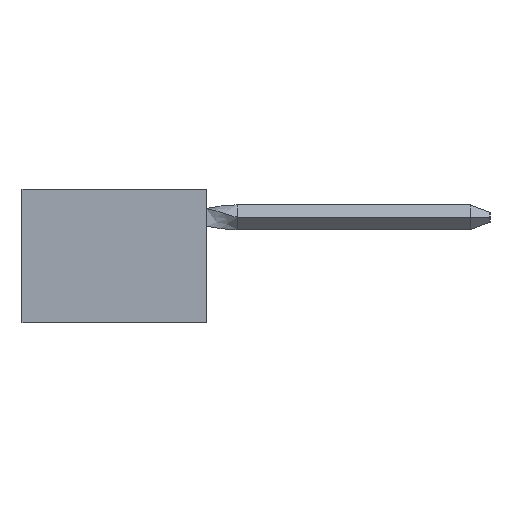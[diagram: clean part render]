
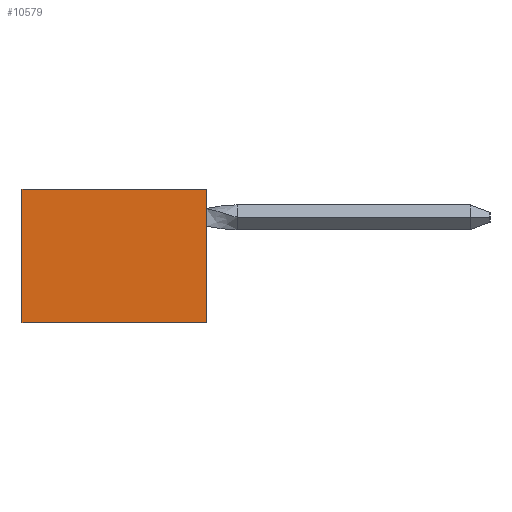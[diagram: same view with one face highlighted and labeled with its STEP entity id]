
A CAD part, left-side view. The second image highlights one B-rep face of the part: STEP entity #10579.
In plain terms, the highlighted planar face has unit normal (-1, 0, 0).
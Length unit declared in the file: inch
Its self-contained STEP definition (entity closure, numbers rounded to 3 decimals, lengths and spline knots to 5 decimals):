
#341 = LINE ( 'NONE', #5239, #14562 ) ;
#389 = LINE ( 'NONE', #11272, #28761 ) ;
#929 = PLANE ( 'NONE',  #28540 ) ;
#1542 = LINE ( 'NONE', #12609, #11297 ) ;
#4967 = VERTEX_POINT ( 'NONE', #35249 ) ;
#5239 = CARTESIAN_POINT ( 'NONE',  ( 0.298, 0., -0.343 ) ) ;
#5421 = EDGE_CURVE ( 'NONE', #27252, #29198, #389, .T. ) ;
#5598 = CARTESIAN_POINT ( 'NONE',  ( 0.298, 0.473, 0. ) ) ;
#7021 = CARTESIAN_POINT ( 'NONE',  ( 0.298, 0., 0. ) ) ;
#7313 = LINE ( 'NONE', #35291, #29466 ) ;
#9545 = EDGE_CURVE ( 'NONE', #16041, #27252, #1542, .T. ) ;
#10579 = ADVANCED_FACE ( 'NONE', ( #16104 ), #929, .F. ) ;
#10687 = DIRECTION ( 'NONE',  ( 0., 0., 1. ) ) ;
#11255 = ORIENTED_EDGE ( 'NONE', *, *, #5421, .T. ) ;
#11272 = CARTESIAN_POINT ( 'NONE',  ( 0.298, 0.473, 0. ) ) ;
#11297 = VECTOR ( 'NONE', #35463, 39.37008 ) ;
#12609 = CARTESIAN_POINT ( 'NONE',  ( 0.298, -0.027, 0. ) ) ;
#13822 = ORIENTED_EDGE ( 'NONE', *, *, #28765, .F. ) ;
#13982 = EDGE_CURVE ( 'NONE', #4967, #16041, #341, .T. ) ;
#14562 = VECTOR ( 'NONE', #10687, 39.37008 ) ;
#15285 = DIRECTION ( 'NONE',  ( 0., 1., 0. ) ) ;
#15472 = ORIENTED_EDGE ( 'NONE', *, *, #9545, .T. ) ;
#16041 = VERTEX_POINT ( 'NONE', #7021 ) ;
#16104 = FACE_OUTER_BOUND ( 'NONE', #16666, .T. ) ;
#16666 = EDGE_LOOP ( 'NONE', ( #29455, #15472, #11255, #13822 ) ) ;
#17948 = CARTESIAN_POINT ( 'NONE',  ( 0.298, -0.027, 0. ) ) ;
#19803 = CARTESIAN_POINT ( 'NONE',  ( 0.298, 0.473, -0.343 ) ) ;
#20989 = DIRECTION ( 'NONE',  ( 0., 0., -1. ) ) ;
#23614 = DIRECTION ( 'NONE',  ( 1., 0., 0. ) ) ;
#27252 = VERTEX_POINT ( 'NONE', #5598 ) ;
#28540 = AXIS2_PLACEMENT_3D ( 'NONE', #17948, #23614, #20989 ) ;
#28761 = VECTOR ( 'NONE', #30932, 39.37008 ) ;
#28765 = EDGE_CURVE ( 'NONE', #4967, #29198, #7313, .T. ) ;
#29198 = VERTEX_POINT ( 'NONE', #19803 ) ;
#29455 = ORIENTED_EDGE ( 'NONE', *, *, #13982, .T. ) ;
#29466 = VECTOR ( 'NONE', #15285, 39.37008 ) ;
#30932 = DIRECTION ( 'NONE',  ( 0., 0., -1. ) ) ;
#35249 = CARTESIAN_POINT ( 'NONE',  ( 0.298, 0., -0.343 ) ) ;
#35291 = CARTESIAN_POINT ( 'NONE',  ( 0.298, 0.473, -0.343 ) ) ;
#35463 = DIRECTION ( 'NONE',  ( 0., 1., 0. ) ) ;
